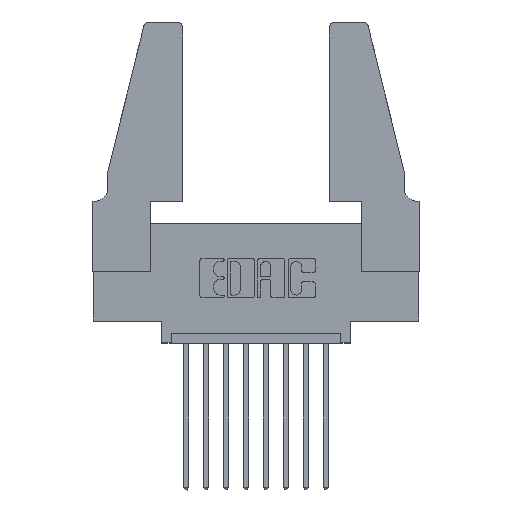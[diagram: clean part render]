
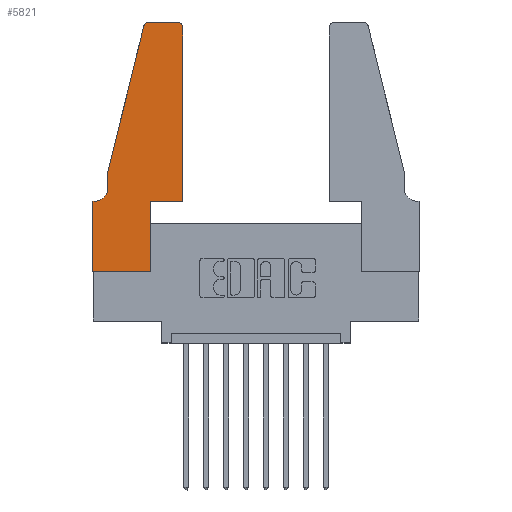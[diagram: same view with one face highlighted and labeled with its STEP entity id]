
A CAD part, top view. The second image highlights one B-rep face of the part: STEP entity #5821.
In plain terms, the highlighted planar face has unit normal (0, 0, 1).
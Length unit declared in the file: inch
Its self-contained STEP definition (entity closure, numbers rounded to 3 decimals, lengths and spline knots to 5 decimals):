
#13 = CARTESIAN_POINT ( 'NONE',  ( 0.2605, 1.25, 0.37 ) ) ;
#54 = CARTESIAN_POINT ( 'NONE',  ( 0., 0., 0.37 ) ) ;
#108 = CARTESIAN_POINT ( 'NONE',  ( 0.25487, 1.22718, 0.37 ) ) ;
#401 = CARTESIAN_POINT ( 'NONE',  ( 0., 0.35, 0.37 ) ) ;
#477 = VERTEX_POINT ( 'NONE', #11880 ) ;
#645 = ORIENTED_EDGE ( 'NONE', *, *, #6191, .T. ) ;
#711 = CARTESIAN_POINT ( 'NONE',  ( 0.4205, 1.22, 0.37 ) ) ;
#734 = ORIENTED_EDGE ( 'NONE', *, *, #12720, .T. ) ;
#962 = DIRECTION ( 'NONE',  ( 1., 0., 0. ) ) ;
#1036 = DIRECTION ( 'NONE',  ( -1., 0., 0. ) ) ;
#1127 = VECTOR ( 'NONE', #10807, 39.37008 ) ;
#1169 = ORIENTED_EDGE ( 'NONE', *, *, #2614, .T. ) ;
#1311 = CARTESIAN_POINT ( 'NONE',  ( 0.2865, 0., 0.37 ) ) ;
#1369 = EDGE_CURVE ( 'NONE', #12821, #10000, #8652, .T. ) ;
#1446 = CIRCLE ( 'NONE', #1789, 0.03 ) ;
#1570 = EDGE_CURVE ( 'NONE', #3611, #12821, #7100, .T. ) ;
#1668 = CARTESIAN_POINT ( 'NONE',  ( 0.4505, 1.22, 0.37 ) ) ;
#1701 = LINE ( 'NONE', #13, #10143 ) ;
#1733 = ORIENTED_EDGE ( 'NONE', *, *, #1570, .T. ) ;
#1789 = AXIS2_PLACEMENT_3D ( 'NONE', #4882, #2748, #12759 ) ;
#1814 = CARTESIAN_POINT ( 'NONE',  ( 0.0755, 0.35, 0.37 ) ) ;
#2160 = AXIS2_PLACEMENT_3D ( 'NONE', #401, #2411, #4348 ) ;
#2191 = VERTEX_POINT ( 'NONE', #9912 ) ;
#2233 = ORIENTED_EDGE ( 'NONE', *, *, #8676, .T. ) ;
#2237 = LINE ( 'NONE', #10485, #10993 ) ;
#2411 = DIRECTION ( 'NONE',  ( 0., 0., 1. ) ) ;
#2417 = AXIS2_PLACEMENT_3D ( 'NONE', #711, #11496, #4634 ) ;
#2429 = CARTESIAN_POINT ( 'NONE',  ( 0., 0., 0.37 ) ) ;
#2488 = ORIENTED_EDGE ( 'NONE', *, *, #11935, .T. ) ;
#2489 = DIRECTION ( 'NONE',  ( -1., 0., 0. ) ) ;
#2513 = VERTEX_POINT ( 'NONE', #2429 ) ;
#2532 = ORIENTED_EDGE ( 'NONE', *, *, #1369, .T. ) ;
#2614 = EDGE_CURVE ( 'NONE', #8588, #2191, #7852, .T. ) ;
#2748 = DIRECTION ( 'NONE',  ( 0., 0., 1. ) ) ;
#3134 = LINE ( 'NONE', #9858, #1127 ) ;
#3454 = ORIENTED_EDGE ( 'NONE', *, *, #3833, .T. ) ;
#3497 = VECTOR ( 'NONE', #9633, 39.37008 ) ;
#3551 = CARTESIAN_POINT ( 'NONE',  ( 0.0055, 0.35, 0.37 ) ) ;
#3611 = VERTEX_POINT ( 'NONE', #5324 ) ;
#3628 = CARTESIAN_POINT ( 'NONE',  ( 0.2865, 0.35, 0.37 ) ) ;
#3667 = VECTOR ( 'NONE', #9112, 39.37008 ) ;
#3833 = EDGE_CURVE ( 'NONE', #9717, #10773, #1446, .T. ) ;
#3993 = LINE ( 'NONE', #54, #3667 ) ;
#4348 = DIRECTION ( 'NONE',  ( 1., 0., 0. ) ) ;
#4508 = DIRECTION ( 'NONE',  ( -0.239, -0.971, 0. ) ) ;
#4634 = DIRECTION ( 'NONE',  ( 1., 0., 0. ) ) ;
#4764 = ORIENTED_EDGE ( 'NONE', *, *, #9575, .T. ) ;
#4815 = LINE ( 'NONE', #7873, #12757 ) ;
#4882 = CARTESIAN_POINT ( 'NONE',  ( 0.284, 1.22, 0.37 ) ) ;
#5066 = CARTESIAN_POINT ( 'NONE',  ( 0.4505, 0.35, 0.37 ) ) ;
#5114 = ORIENTED_EDGE ( 'NONE', *, *, #5315, .T. ) ;
#5315 = EDGE_CURVE ( 'NONE', #12778, #11648, #4815, .T. ) ;
#5324 = CARTESIAN_POINT ( 'NONE',  ( 0.0755, 0.5, 0.37 ) ) ;
#5821 = ADVANCED_FACE ( 'NONE', ( #7427 ), #12367, .T. ) ;
#6191 = EDGE_CURVE ( 'NONE', #2513, #8588, #3993, .T. ) ;
#6242 = EDGE_LOOP ( 'NONE', ( #4764, #3454, #8447, #1733, #2532, #2488, #2233, #645, #1169, #734, #5114, #8479 ) ) ;
#6264 = DIRECTION ( 'NONE',  ( 0., 0., -1. ) ) ;
#6795 = EDGE_CURVE ( 'NONE', #10773, #3611, #2237, .T. ) ;
#6952 = VECTOR ( 'NONE', #2489, 39.37008 ) ;
#7100 = LINE ( 'NONE', #9645, #10381 ) ;
#7391 = CARTESIAN_POINT ( 'NONE',  ( 0.0055, 0.42, 0.37 ) ) ;
#7425 = EDGE_CURVE ( 'NONE', #11648, #8336, #10361, .T. ) ;
#7427 = FACE_OUTER_BOUND ( 'NONE', #6242, .T. ) ;
#7689 = LINE ( 'NONE', #8007, #9403 ) ;
#7852 = LINE ( 'NONE', #3628, #3497 ) ;
#7873 = CARTESIAN_POINT ( 'NONE',  ( 0.4505, 0.35, 0.37 ) ) ;
#8007 = CARTESIAN_POINT ( 'NONE',  ( 0.4505, 0.35, 0.37 ) ) ;
#8336 = VERTEX_POINT ( 'NONE', #10090 ) ;
#8447 = ORIENTED_EDGE ( 'NONE', *, *, #6795, .T. ) ;
#8479 = ORIENTED_EDGE ( 'NONE', *, *, #7425, .T. ) ;
#8588 = VERTEX_POINT ( 'NONE', #1311 ) ;
#8652 = CIRCLE ( 'NONE', #10456, 0.07 ) ;
#8676 = EDGE_CURVE ( 'NONE', #477, #2513, #3134, .T. ) ;
#8830 = DIRECTION ( 'NONE',  ( 0., 1., 0. ) ) ;
#8984 = CARTESIAN_POINT ( 'NONE',  ( 0.0755, 0.42, 0.37 ) ) ;
#9112 = DIRECTION ( 'NONE',  ( 1., 0., 0. ) ) ;
#9403 = VECTOR ( 'NONE', #962, 39.37008 ) ;
#9575 = EDGE_CURVE ( 'NONE', #8336, #9717, #1701, .T. ) ;
#9589 = LINE ( 'NONE', #1814, #6952 ) ;
#9633 = DIRECTION ( 'NONE',  ( 0., 1., 0. ) ) ;
#9645 = CARTESIAN_POINT ( 'NONE',  ( 0.0755, 0.5, 0.37 ) ) ;
#9717 = VERTEX_POINT ( 'NONE', #12923 ) ;
#9858 = CARTESIAN_POINT ( 'NONE',  ( 0., 0., 0.37 ) ) ;
#9912 = CARTESIAN_POINT ( 'NONE',  ( 0.2865, 0.35, 0.37 ) ) ;
#10000 = VERTEX_POINT ( 'NONE', #3551 ) ;
#10090 = CARTESIAN_POINT ( 'NONE',  ( 0.4205, 1.25, 0.37 ) ) ;
#10143 = VECTOR ( 'NONE', #1036, 39.37008 ) ;
#10360 = DIRECTION ( 'NONE',  ( -1., 0., 0. ) ) ;
#10361 = CIRCLE ( 'NONE', #2417, 0.03 ) ;
#10381 = VECTOR ( 'NONE', #12693, 39.37008 ) ;
#10456 = AXIS2_PLACEMENT_3D ( 'NONE', #7391, #6264, #10360 ) ;
#10485 = CARTESIAN_POINT ( 'NONE',  ( 0.0755, 0.5, 0.37 ) ) ;
#10773 = VERTEX_POINT ( 'NONE', #108 ) ;
#10807 = DIRECTION ( 'NONE',  ( 0., -1., 0. ) ) ;
#10993 = VECTOR ( 'NONE', #4508, 39.37008 ) ;
#11496 = DIRECTION ( 'NONE',  ( 0., 0., 1. ) ) ;
#11648 = VERTEX_POINT ( 'NONE', #1668 ) ;
#11880 = CARTESIAN_POINT ( 'NONE',  ( 0., 0.35, 0.37 ) ) ;
#11935 = EDGE_CURVE ( 'NONE', #10000, #477, #9589, .T. ) ;
#12367 = PLANE ( 'NONE',  #2160 ) ;
#12693 = DIRECTION ( 'NONE',  ( 0., -1., 0. ) ) ;
#12720 = EDGE_CURVE ( 'NONE', #2191, #12778, #7689, .T. ) ;
#12757 = VECTOR ( 'NONE', #8830, 39.37008 ) ;
#12759 = DIRECTION ( 'NONE',  ( 1., 0., 0. ) ) ;
#12778 = VERTEX_POINT ( 'NONE', #5066 ) ;
#12821 = VERTEX_POINT ( 'NONE', #8984 ) ;
#12923 = CARTESIAN_POINT ( 'NONE',  ( 0.284, 1.25, 0.37 ) ) ;
